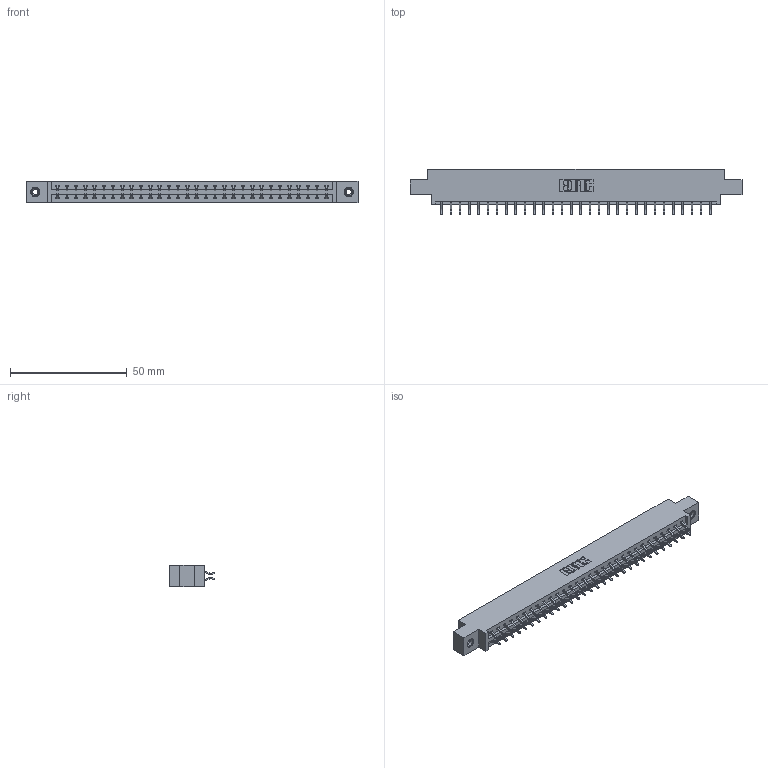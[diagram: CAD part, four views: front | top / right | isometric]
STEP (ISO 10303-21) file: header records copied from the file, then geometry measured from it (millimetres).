
FILE_DESCRIPTION (( 'STEP AP203' ), '1' );
FILE_NAME ('387-060-556-808.STEP', '2019-10-19T14:06:25', ( '' ), ( '' ), 'SwSTEP 2.0', 'SolidWorks 2016', '' );
FILE_SCHEMA (( 'CONFIG_CONTROL_DESIGN' ));
Length unit declared in the file: inch
Products named in the file (4): 337 Part_0.170 Offset - 0.156 Dia-TI; 345-250-001_345-250-003-102; 345-292-001_556 Tail; 387-060-556-808
Assembly tree (63 placements, depth 2):
  387-060-556-808
    337 Part_0.170 Offset - 0.156 Dia-TI
    345-292-001_556 Tail  x60
    345-250-001_345-250-003-102  x2
Bounding box: 141.88 x 19.57 x 9.4 mm (x, y, z)
Volume: 14666.8 mm3; surface area: 16532.7 mm2
Topology: 63 solids, 63 shells, 3778 faces, 11199 edges, 7378 vertices
Faces by surface type: plane 2626, cylinder 1136, cone 12, torus 4
Entity records: 26350 total; most frequent: CARTESIAN_POINT 4445, ORIENTED_EDGE 4362, DIRECTION 3823, EDGE_CURVE 2181, LINE 2025, VECTOR 2025, VERTEX_POINT 1448, AXIS2_PLACEMENT_3D 899
